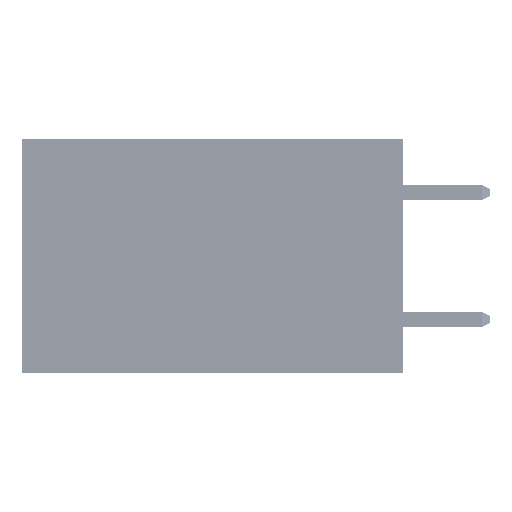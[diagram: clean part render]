
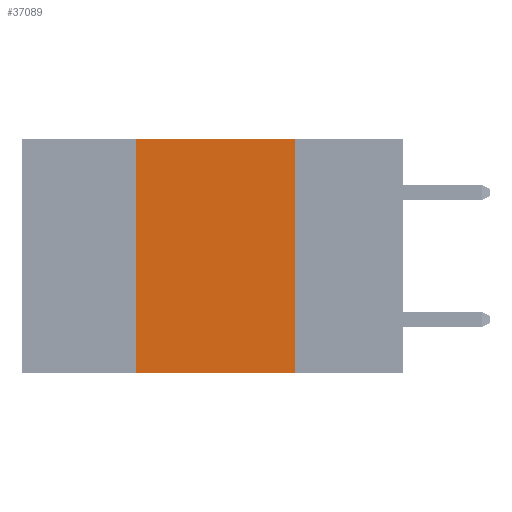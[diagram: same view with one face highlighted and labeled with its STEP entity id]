
A CAD part, left-side view. The second image highlights one B-rep face of the part: STEP entity #37089.
In plain terms, the highlighted planar face has unit normal (-1, 0, 0).
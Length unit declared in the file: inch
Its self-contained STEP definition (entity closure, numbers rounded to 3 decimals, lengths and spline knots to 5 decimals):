
#393 = DIRECTION ( 'NONE',  ( 0., -1., 0. ) ) ;
#1329 = DIRECTION ( 'NONE',  ( 0., 0., -1. ) ) ;
#3539 = AXIS2_PLACEMENT_3D ( 'NONE', #32922, #47894, #10093 ) ;
#6001 = LINE ( 'NONE', #31225, #37659 ) ;
#8784 = CARTESIAN_POINT ( 'NONE',  ( 0., 0.42, -0.37 ) ) ;
#10093 = DIRECTION ( 'NONE',  ( 0., 0., -1. ) ) ;
#11614 = ORIENTED_EDGE ( 'NONE', *, *, #29487, .F. ) ;
#12216 = DIRECTION ( 'NONE',  ( 0., 0., 1. ) ) ;
#12260 = CARTESIAN_POINT ( 'NONE',  ( 0., 0.6, 0. ) ) ;
#15110 = ORIENTED_EDGE ( 'NONE', *, *, #18447, .T. ) ;
#15209 = CARTESIAN_POINT ( 'NONE',  ( 0., 0.17, 0. ) ) ;
#17299 = VECTOR ( 'NONE', #393, 39.37008 ) ;
#18447 = EDGE_CURVE ( 'NONE', #27895, #48125, #29287, .T. ) ;
#23366 = VECTOR ( 'NONE', #12216, 39.37008 ) ;
#23712 = EDGE_LOOP ( 'NONE', ( #37638, #11614, #36813, #15110 ) ) ;
#24342 = FACE_OUTER_BOUND ( 'NONE', #23712, .T. ) ;
#27895 = VERTEX_POINT ( 'NONE', #8784 ) ;
#28429 = PLANE ( 'NONE',  #3539 ) ;
#28668 = CARTESIAN_POINT ( 'NONE',  ( 0., 0.6, -0.37 ) ) ;
#29287 = LINE ( 'NONE', #28668, #44828 ) ;
#29487 = EDGE_CURVE ( 'NONE', #45875, #44226, #38234, .T. ) ;
#31225 = CARTESIAN_POINT ( 'NONE',  ( 0., 0.17, 0. ) ) ;
#32512 = DIRECTION ( 'NONE',  ( 0., -1., 0. ) ) ;
#32922 = CARTESIAN_POINT ( 'NONE',  ( 0., 0.6, 0. ) ) ;
#33152 = CARTESIAN_POINT ( 'NONE',  ( 0., 0.17, -0.37 ) ) ;
#33488 = CARTESIAN_POINT ( 'NONE',  ( 0., 0.42, 0. ) ) ;
#35068 = CARTESIAN_POINT ( 'NONE',  ( 0., 0.42, 0. ) ) ;
#35690 = EDGE_CURVE ( 'NONE', #44226, #48125, #6001, .T. ) ;
#36813 = ORIENTED_EDGE ( 'NONE', *, *, #41063, .F. ) ;
#37089 = ADVANCED_FACE ( 'NONE', ( #24342 ), #28429, .F. ) ;
#37638 = ORIENTED_EDGE ( 'NONE', *, *, #35690, .F. ) ;
#37659 = VECTOR ( 'NONE', #1329, 39.37008 ) ;
#38234 = LINE ( 'NONE', #12260, #17299 ) ;
#41063 = EDGE_CURVE ( 'NONE', #27895, #45875, #42463, .T. ) ;
#42463 = LINE ( 'NONE', #35068, #23366 ) ;
#44226 = VERTEX_POINT ( 'NONE', #15209 ) ;
#44828 = VECTOR ( 'NONE', #32512, 39.37008 ) ;
#45875 = VERTEX_POINT ( 'NONE', #33488 ) ;
#47894 = DIRECTION ( 'NONE',  ( 1., 0., 0. ) ) ;
#48125 = VERTEX_POINT ( 'NONE', #33152 ) ;
